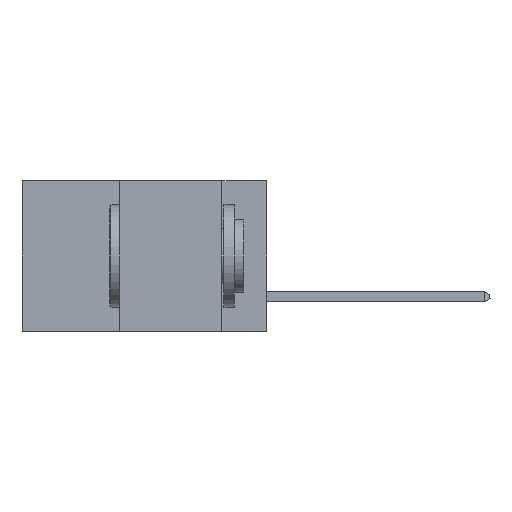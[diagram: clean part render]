
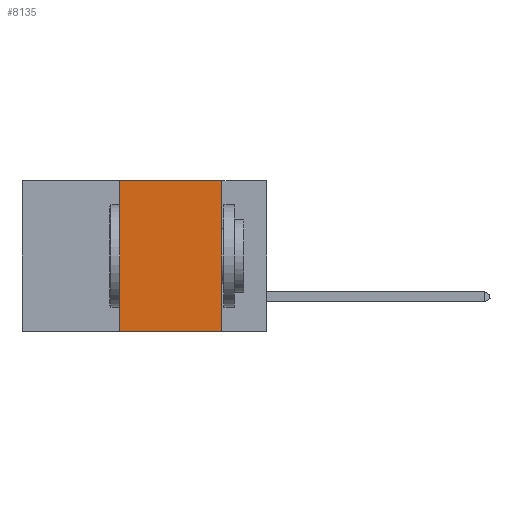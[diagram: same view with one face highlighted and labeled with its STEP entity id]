
A CAD part, left-side view. The second image highlights one B-rep face of the part: STEP entity #8135.
In plain terms, the highlighted planar face has unit normal (-1, 0, 0).
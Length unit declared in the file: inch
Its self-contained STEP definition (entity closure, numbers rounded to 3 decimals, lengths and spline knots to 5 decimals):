
#565 = LINE ( 'NONE', #43348, #25143 ) ;
#2060 = DIRECTION ( 'NONE',  ( 1., 0., 0. ) ) ;
#2359 = CARTESIAN_POINT ( 'NONE',  ( 0., 0.11, 0. ) ) ;
#3762 = VECTOR ( 'NONE', #46643, 39.37008 ) ;
#6140 = CARTESIAN_POINT ( 'NONE',  ( 0., 0.6, 0. ) ) ;
#6354 = CARTESIAN_POINT ( 'NONE',  ( 0., 0.36, -0.37 ) ) ;
#6617 = EDGE_CURVE ( 'NONE', #17733, #15770, #22474, .T. ) ;
#7644 = VECTOR ( 'NONE', #41988, 39.37008 ) ;
#8135 = ADVANCED_FACE ( 'NONE', ( #22881 ), #28861, .F. ) ;
#8156 = VERTEX_POINT ( 'NONE', #17583 ) ;
#9574 = DIRECTION ( 'NONE',  ( 0., 0., -1. ) ) ;
#9988 = ORIENTED_EDGE ( 'NONE', *, *, #17637, .F. ) ;
#11145 = CARTESIAN_POINT ( 'NONE',  ( 0., 0.11, -0.37 ) ) ;
#12228 = EDGE_LOOP ( 'NONE', ( #33042, #9988, #27536, #46038 ) ) ;
#12890 = LINE ( 'NONE', #45596, #7644 ) ;
#14709 = EDGE_CURVE ( 'NONE', #8156, #20533, #37374, .T. ) ;
#15770 = VERTEX_POINT ( 'NONE', #21037 ) ;
#17190 = DIRECTION ( 'NONE',  ( 0., -1., 0. ) ) ;
#17583 = CARTESIAN_POINT ( 'NONE',  ( 0., 0.11, 0. ) ) ;
#17637 = EDGE_CURVE ( 'NONE', #15770, #8156, #12890, .T. ) ;
#17733 = VERTEX_POINT ( 'NONE', #6354 ) ;
#18928 = EDGE_CURVE ( 'NONE', #17733, #20533, #565, .T. ) ;
#20533 = VERTEX_POINT ( 'NONE', #11145 ) ;
#21037 = CARTESIAN_POINT ( 'NONE',  ( 0., 0.36, 0. ) ) ;
#22474 = LINE ( 'NONE', #39282, #3762 ) ;
#22881 = FACE_OUTER_BOUND ( 'NONE', #12228, .T. ) ;
#23877 = VECTOR ( 'NONE', #28503, 39.37008 ) ;
#25143 = VECTOR ( 'NONE', #17190, 39.37008 ) ;
#27536 = ORIENTED_EDGE ( 'NONE', *, *, #6617, .F. ) ;
#28503 = DIRECTION ( 'NONE',  ( 0., 0., -1. ) ) ;
#28861 = PLANE ( 'NONE',  #46937 ) ;
#33042 = ORIENTED_EDGE ( 'NONE', *, *, #14709, .F. ) ;
#37374 = LINE ( 'NONE', #2359, #23877 ) ;
#39282 = CARTESIAN_POINT ( 'NONE',  ( 0., 0.36, 0. ) ) ;
#41988 = DIRECTION ( 'NONE',  ( 0., -1., 0. ) ) ;
#43348 = CARTESIAN_POINT ( 'NONE',  ( 0., 0.6, -0.37 ) ) ;
#45596 = CARTESIAN_POINT ( 'NONE',  ( 0., 0.6, 0. ) ) ;
#46038 = ORIENTED_EDGE ( 'NONE', *, *, #18928, .T. ) ;
#46643 = DIRECTION ( 'NONE',  ( 0., 0., 1. ) ) ;
#46937 = AXIS2_PLACEMENT_3D ( 'NONE', #6140, #2060, #9574 ) ;
